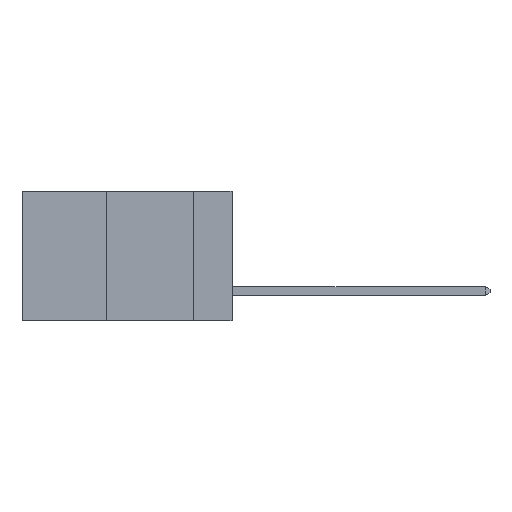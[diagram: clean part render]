
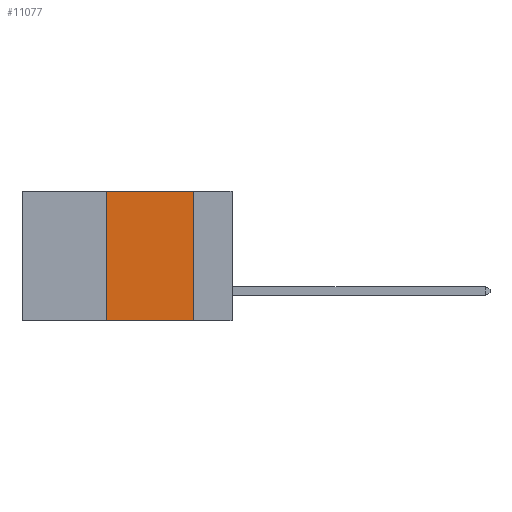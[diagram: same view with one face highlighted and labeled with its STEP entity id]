
A CAD part, left-side view. The second image highlights one B-rep face of the part: STEP entity #11077.
In plain terms, the highlighted planar face has unit normal (-1, 0, 0).
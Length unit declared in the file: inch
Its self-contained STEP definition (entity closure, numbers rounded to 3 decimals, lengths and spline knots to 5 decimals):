
#524 = CARTESIAN_POINT ( 'NONE',  ( 0., 0.36, -0.37 ) ) ;
#867 = ORIENTED_EDGE ( 'NONE', *, *, #5569, .F. ) ;
#1746 = PLANE ( 'NONE',  #2047 ) ;
#1818 = VERTEX_POINT ( 'NONE', #524 ) ;
#2047 = AXIS2_PLACEMENT_3D ( 'NONE', #2972, #10336, #4096 ) ;
#2821 = VERTEX_POINT ( 'NONE', #12118 ) ;
#2972 = CARTESIAN_POINT ( 'NONE',  ( 0., 0.6, 0. ) ) ;
#3255 = ORIENTED_EDGE ( 'NONE', *, *, #6246, .T. ) ;
#3511 = CARTESIAN_POINT ( 'NONE',  ( 0., 0.11, -0.37 ) ) ;
#3653 = VERTEX_POINT ( 'NONE', #6171 ) ;
#3674 = CARTESIAN_POINT ( 'NONE',  ( 0., 0.6, 0. ) ) ;
#4096 = DIRECTION ( 'NONE',  ( 0., 0., -1. ) ) ;
#4483 = FACE_OUTER_BOUND ( 'NONE', #5462, .T. ) ;
#4549 = VECTOR ( 'NONE', #7950, 39.37008 ) ;
#4877 = DIRECTION ( 'NONE',  ( 0., 0., -1. ) ) ;
#5274 = LINE ( 'NONE', #5283, #7756 ) ;
#5283 = CARTESIAN_POINT ( 'NONE',  ( 0., 0.36, 0. ) ) ;
#5462 = EDGE_LOOP ( 'NONE', ( #867, #12634, #7946, #3255 ) ) ;
#5569 = EDGE_CURVE ( 'NONE', #2821, #9576, #11893, .T. ) ;
#6171 = CARTESIAN_POINT ( 'NONE',  ( 0., 0.36, 0. ) ) ;
#6246 = EDGE_CURVE ( 'NONE', #1818, #9576, #11728, .T. ) ;
#6924 = CARTESIAN_POINT ( 'NONE',  ( 0., 0.11, 0. ) ) ;
#7756 = VECTOR ( 'NONE', #10394, 39.37008 ) ;
#7946 = ORIENTED_EDGE ( 'NONE', *, *, #8359, .F. ) ;
#7950 = DIRECTION ( 'NONE',  ( 0., -1., 0. ) ) ;
#8359 = EDGE_CURVE ( 'NONE', #1818, #3653, #5274, .T. ) ;
#9183 = EDGE_CURVE ( 'NONE', #3653, #2821, #12353, .T. ) ;
#9245 = VECTOR ( 'NONE', #4877, 39.37008 ) ;
#9384 = VECTOR ( 'NONE', #12044, 39.37008 ) ;
#9576 = VERTEX_POINT ( 'NONE', #3511 ) ;
#10336 = DIRECTION ( 'NONE',  ( 1., 0., 0. ) ) ;
#10394 = DIRECTION ( 'NONE',  ( 0., 0., 1. ) ) ;
#11077 = ADVANCED_FACE ( 'NONE', ( #4483 ), #1746, .F. ) ;
#11084 = CARTESIAN_POINT ( 'NONE',  ( 0., 0.6, -0.37 ) ) ;
#11728 = LINE ( 'NONE', #11084, #9384 ) ;
#11893 = LINE ( 'NONE', #6924, #9245 ) ;
#12044 = DIRECTION ( 'NONE',  ( 0., -1., 0. ) ) ;
#12118 = CARTESIAN_POINT ( 'NONE',  ( 0., 0.11, 0. ) ) ;
#12353 = LINE ( 'NONE', #3674, #4549 ) ;
#12634 = ORIENTED_EDGE ( 'NONE', *, *, #9183, .F. ) ;
